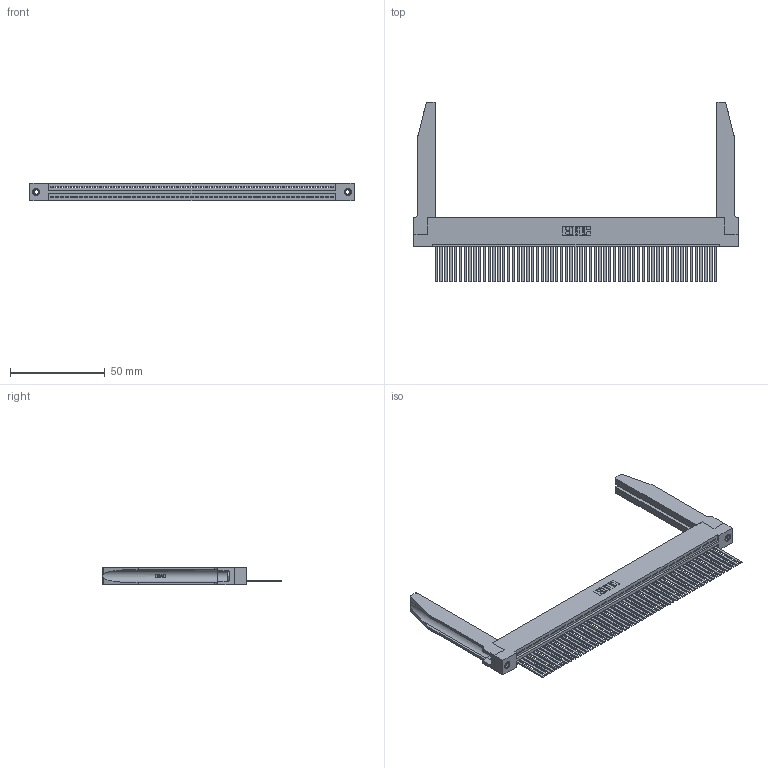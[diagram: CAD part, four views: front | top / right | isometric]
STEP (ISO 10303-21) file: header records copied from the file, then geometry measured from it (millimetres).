
FILE_DESCRIPTION (( 'STEP AP203' ), '1' );
FILE_NAME ('345-059-544-178.STEP', '2019-10-10T20:44:32', ( '' ), ( '' ), 'SwSTEP 2.0', 'SolidWorks 2016', '' );
FILE_SCHEMA (( 'CONFIG_CONTROL_DESIGN' ));
Length unit declared in the file: inch
Products named in the file (5): 345-292-001_345-293-144; 345-250-001_345-250-001-102; 345-059-544-178; 345-220-078_345-220-078; 345 Part_Flush Mounting Lugs - 0.156 Dia-TH
Assembly tree (64 placements, depth 2):
  345-059-544-178
    345 Part_Flush Mounting Lugs - 0.156 Dia-TH
    345-292-001_345-293-144  x59
    345-250-001_345-250-001-102  x2
    345-220-078_345-220-078  x2
Bounding box: 171.09 x 94.92 x 9.4 mm (x, y, z)
Volume: 24843.8 mm3; surface area: 31816.8 mm2
Topology: 64 solids, 64 shells, 3428 faces, 10271 edges, 6758 vertices
Faces by surface type: plane 2346, cylinder 1030, bspline 36, cone 12, torus 4
Entity records: 46672 total; most frequent: CARTESIAN_POINT 8980, ORIENTED_EDGE 7870, DIRECTION 6823, EDGE_CURVE 3935, LINE 3477, VECTOR 3477, VERTEX_POINT 2616, AXIS2_PLACEMENT_3D 1673
